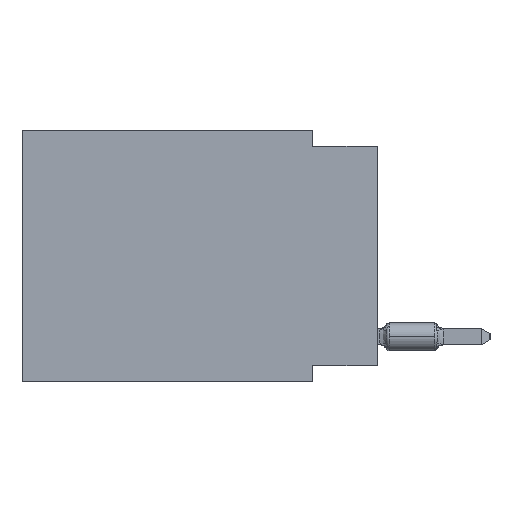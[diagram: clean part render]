
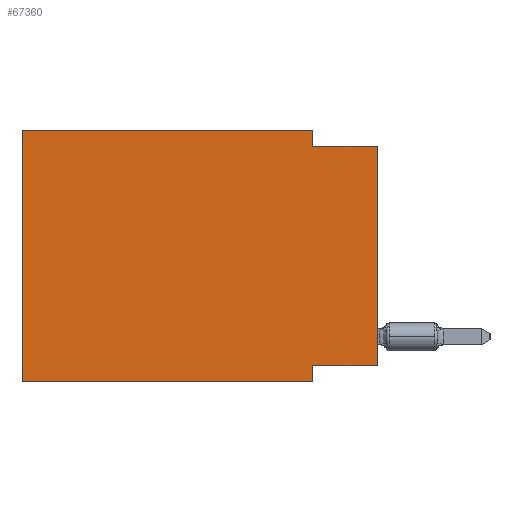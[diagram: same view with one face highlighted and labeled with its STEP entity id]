
A CAD part, left-side view. The second image highlights one B-rep face of the part: STEP entity #67360.
In plain terms, the highlighted planar face has unit normal (-1, 0, 0).
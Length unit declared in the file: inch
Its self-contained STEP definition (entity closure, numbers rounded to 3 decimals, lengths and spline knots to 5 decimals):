
#119 = EDGE_CURVE ( 'NONE', #21196, #28683, #22094, .T. ) ;
#831 = CARTESIAN_POINT ( 'NONE',  ( 0., 0.55, 0. ) ) ;
#1405 = VERTEX_POINT ( 'NONE', #49016 ) ;
#2489 = LINE ( 'NONE', #24060, #45038 ) ;
#4622 = EDGE_CURVE ( 'NONE', #38203, #29459, #46141, .T. ) ;
#4905 = VERTEX_POINT ( 'NONE', #8716 ) ;
#5436 = LINE ( 'NONE', #9959, #41362 ) ;
#5587 = CARTESIAN_POINT ( 'NONE',  ( 0., 0.55, 0. ) ) ;
#6396 = VECTOR ( 'NONE', #27344, 39.37008 ) ;
#8716 = CARTESIAN_POINT ( 'NONE',  ( 0., 0.55, -0.39 ) ) ;
#9737 = EDGE_CURVE ( 'NONE', #4905, #50484, #5436, .T. ) ;
#9959 = CARTESIAN_POINT ( 'NONE',  ( 0., 0.55, 0. ) ) ;
#10108 = PLANE ( 'NONE',  #27319 ) ;
#10483 = ORIENTED_EDGE ( 'NONE', *, *, #4622, .F. ) ;
#12313 = CARTESIAN_POINT ( 'NONE',  ( 0., 0.1, -0.39 ) ) ;
#12463 = EDGE_LOOP ( 'NONE', ( #23189, #10483, #38468, #37811, #59062, #15751, #56033, #24158 ) ) ;
#12472 = EDGE_CURVE ( 'NONE', #4905, #28683, #47672, .T. ) ;
#13574 = VECTOR ( 'NONE', #22037, 39.37008 ) ;
#13829 = CARTESIAN_POINT ( 'NONE',  ( 0., 0., 0. ) ) ;
#13924 = VERTEX_POINT ( 'NONE', #28141 ) ;
#14502 = CARTESIAN_POINT ( 'NONE',  ( 0., 0.55, -0.39 ) ) ;
#15751 = ORIENTED_EDGE ( 'NONE', *, *, #12472, .T. ) ;
#19940 = CARTESIAN_POINT ( 'NONE',  ( 0., 0.1, -0.365 ) ) ;
#20894 = DIRECTION ( 'NONE',  ( 0., 0., -1. ) ) ;
#21196 = VERTEX_POINT ( 'NONE', #19940 ) ;
#22037 = DIRECTION ( 'NONE',  ( 0., -1., 0. ) ) ;
#22094 = LINE ( 'NONE', #12313, #6396 ) ;
#23189 = ORIENTED_EDGE ( 'NONE', *, *, #37338, .T. ) ;
#23671 = EDGE_CURVE ( 'NONE', #50484, #13924, #37779, .T. ) ;
#24060 = CARTESIAN_POINT ( 'NONE',  ( 0., 0.1, 0. ) ) ;
#24158 = ORIENTED_EDGE ( 'NONE', *, *, #61506, .F. ) ;
#25174 = CARTESIAN_POINT ( 'NONE',  ( 0., 0., -0.025 ) ) ;
#25932 = CARTESIAN_POINT ( 'NONE',  ( 0., 0., -0.365 ) ) ;
#27319 = AXIS2_PLACEMENT_3D ( 'NONE', #5587, #57915, #20894 ) ;
#27344 = DIRECTION ( 'NONE',  ( 0., 0., -1. ) ) ;
#28141 = CARTESIAN_POINT ( 'NONE',  ( 0., 0.1, 0. ) ) ;
#28229 = EDGE_CURVE ( 'NONE', #13924, #38203, #2489, .T. ) ;
#28683 = VERTEX_POINT ( 'NONE', #35515 ) ;
#29355 = CARTESIAN_POINT ( 'NONE',  ( 0., 0., -0.025 ) ) ;
#29459 = VERTEX_POINT ( 'NONE', #29355 ) ;
#29777 = LINE ( 'NONE', #25932, #51909 ) ;
#31220 = DIRECTION ( 'NONE',  ( 0., 0., 1. ) ) ;
#35129 = LINE ( 'NONE', #13829, #68555 ) ;
#35515 = CARTESIAN_POINT ( 'NONE',  ( 0., 0.1, -0.39 ) ) ;
#36276 = FACE_OUTER_BOUND ( 'NONE', #12463, .T. ) ;
#37338 = EDGE_CURVE ( 'NONE', #1405, #29459, #35129, .T. ) ;
#37779 = LINE ( 'NONE', #831, #13574 ) ;
#37811 = ORIENTED_EDGE ( 'NONE', *, *, #23671, .F. ) ;
#38203 = VERTEX_POINT ( 'NONE', #46147 ) ;
#38468 = ORIENTED_EDGE ( 'NONE', *, *, #28229, .F. ) ;
#41362 = VECTOR ( 'NONE', #31220, 39.37008 ) ;
#44360 = DIRECTION ( 'NONE',  ( 0., 0., 1. ) ) ;
#45038 = VECTOR ( 'NONE', #66297, 39.37008 ) ;
#46141 = LINE ( 'NONE', #25174, #63170 ) ;
#46147 = CARTESIAN_POINT ( 'NONE',  ( 0., 0.1, -0.025 ) ) ;
#47263 = DIRECTION ( 'NONE',  ( 0., 1., 0. ) ) ;
#47672 = LINE ( 'NONE', #14502, #49224 ) ;
#49016 = CARTESIAN_POINT ( 'NONE',  ( 0., 0., -0.365 ) ) ;
#49224 = VECTOR ( 'NONE', #61948, 39.37008 ) ;
#50484 = VERTEX_POINT ( 'NONE', #55670 ) ;
#51909 = VECTOR ( 'NONE', #47263, 39.37008 ) ;
#55670 = CARTESIAN_POINT ( 'NONE',  ( 0., 0.55, 0. ) ) ;
#56033 = ORIENTED_EDGE ( 'NONE', *, *, #119, .F. ) ;
#57915 = DIRECTION ( 'NONE',  ( 1., 0., 0. ) ) ;
#59062 = ORIENTED_EDGE ( 'NONE', *, *, #9737, .F. ) ;
#61506 = EDGE_CURVE ( 'NONE', #1405, #21196, #29777, .T. ) ;
#61948 = DIRECTION ( 'NONE',  ( 0., -1., 0. ) ) ;
#63170 = VECTOR ( 'NONE', #67757, 39.37008 ) ;
#66297 = DIRECTION ( 'NONE',  ( 0., 0., -1. ) ) ;
#67360 = ADVANCED_FACE ( 'NONE', ( #36276 ), #10108, .F. ) ;
#67757 = DIRECTION ( 'NONE',  ( 0., -1., 0. ) ) ;
#68555 = VECTOR ( 'NONE', #44360, 39.37008 ) ;
